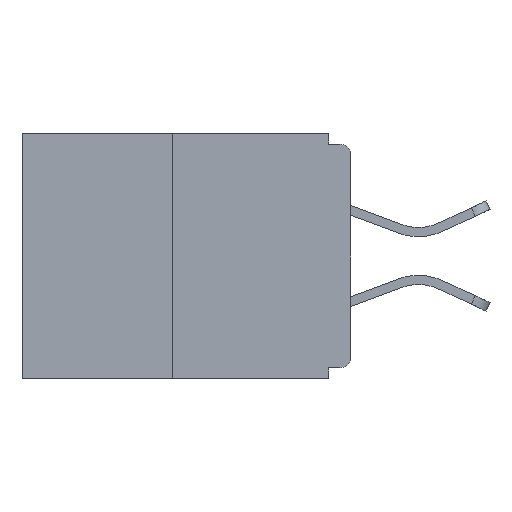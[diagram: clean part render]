
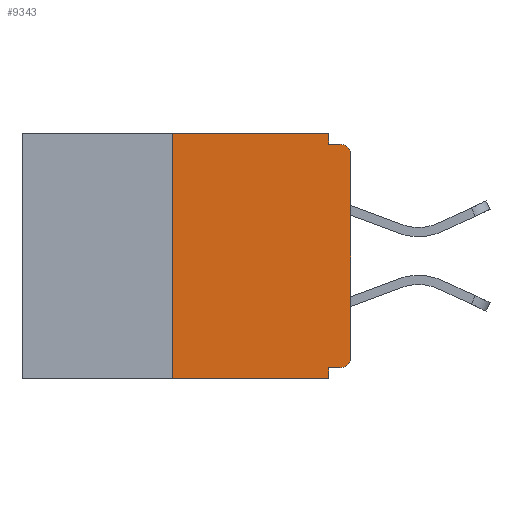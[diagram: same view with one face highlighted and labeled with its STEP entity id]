
A CAD part, left-side view. The second image highlights one B-rep face of the part: STEP entity #9343.
In plain terms, the highlighted planar face has unit normal (-1, 0, 0).
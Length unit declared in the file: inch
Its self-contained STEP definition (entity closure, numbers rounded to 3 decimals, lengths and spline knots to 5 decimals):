
#34 = DIRECTION ( 'NONE',  ( 0., -1., 0. ) ) ;
#90 = ORIENTED_EDGE ( 'NONE', *, *, #9702, .T. ) ;
#694 = CIRCLE ( 'NONE', #2859, 0.015 ) ;
#905 = FACE_OUTER_BOUND ( 'NONE', #6309, .T. ) ;
#1050 = VECTOR ( 'NONE', #14594, 39.37008 ) ;
#1052 = DIRECTION ( 'NONE',  ( 0., -1., 0. ) ) ;
#1120 = VECTOR ( 'NONE', #1052, 39.37008 ) ;
#1260 = VECTOR ( 'NONE', #14195, 39.37008 ) ;
#1294 = AXIS2_PLACEMENT_3D ( 'NONE', #4451, #4503, #5705 ) ;
#1401 = CARTESIAN_POINT ( 'NONE',  ( 0., 0.015, -0.03 ) ) ;
#1433 = LINE ( 'NONE', #3499, #1260 ) ;
#1468 = EDGE_CURVE ( 'NONE', #8898, #9207, #5351, .T. ) ;
#1534 = CIRCLE ( 'NONE', #13776, 0.015 ) ;
#1638 = CARTESIAN_POINT ( 'NONE',  ( 0., 0.015, -0.015 ) ) ;
#1789 = CARTESIAN_POINT ( 'NONE',  ( 0., 0.031, 0. ) ) ;
#1922 = VERTEX_POINT ( 'NONE', #9896 ) ;
#1983 = VECTOR ( 'NONE', #34, 39.37008 ) ;
#2243 = LINE ( 'NONE', #13547, #11268 ) ;
#2253 = ORIENTED_EDGE ( 'NONE', *, *, #13000, .F. ) ;
#2496 = EDGE_CURVE ( 'NONE', #8124, #4469, #1433, .T. ) ;
#2743 = ORIENTED_EDGE ( 'NONE', *, *, #12982, .F. ) ;
#2766 = CARTESIAN_POINT ( 'NONE',  ( 0., 0., 0. ) ) ;
#2859 = AXIS2_PLACEMENT_3D ( 'NONE', #1401, #3673, #8273 ) ;
#3013 = VECTOR ( 'NONE', #8521, 39.37008 ) ;
#3152 = ORIENTED_EDGE ( 'NONE', *, *, #2496, .F. ) ;
#3384 = CARTESIAN_POINT ( 'NONE',  ( 0., 0., -0.313 ) ) ;
#3420 = ORIENTED_EDGE ( 'NONE', *, *, #10922, .T. ) ;
#3435 = PLANE ( 'NONE',  #1294 ) ;
#3499 = CARTESIAN_POINT ( 'NONE',  ( 0., 0., -0.328 ) ) ;
#3620 = CARTESIAN_POINT ( 'NONE',  ( 0., 0.031, -0.343 ) ) ;
#3673 = DIRECTION ( 'NONE',  ( -1., 0., 0. ) ) ;
#3739 = ORIENTED_EDGE ( 'NONE', *, *, #1468, .F. ) ;
#4188 = EDGE_CURVE ( 'NONE', #8089, #10902, #6366, .T. ) ;
#4451 = CARTESIAN_POINT ( 'NONE',  ( 0., 0.46, 0. ) ) ;
#4469 = VERTEX_POINT ( 'NONE', #5397 ) ;
#4503 = DIRECTION ( 'NONE',  ( 1., 0., 0. ) ) ;
#4775 = DIRECTION ( 'NONE',  ( -1., 0., 0. ) ) ;
#5178 = CARTESIAN_POINT ( 'NONE',  ( 0., 0.031, 0. ) ) ;
#5351 = LINE ( 'NONE', #10404, #1120 ) ;
#5397 = CARTESIAN_POINT ( 'NONE',  ( 0., 0.031, -0.328 ) ) ;
#5651 = ORIENTED_EDGE ( 'NONE', *, *, #4188, .T. ) ;
#5667 = CARTESIAN_POINT ( 'NONE',  ( 0., 0., -0.03 ) ) ;
#5705 = DIRECTION ( 'NONE',  ( 0., 0., -1. ) ) ;
#6140 = CARTESIAN_POINT ( 'NONE',  ( 0., 0., -0.015 ) ) ;
#6309 = EDGE_LOOP ( 'NONE', ( #3739, #9972, #3420, #2743, #3152, #9008, #5651, #90, #2253, #8982 ) ) ;
#6366 = LINE ( 'NONE', #2766, #7252 ) ;
#6676 = CARTESIAN_POINT ( 'NONE',  ( 0., 0.25, 0. ) ) ;
#7252 = VECTOR ( 'NONE', #12063, 39.37008 ) ;
#7277 = LINE ( 'NONE', #5178, #1050 ) ;
#7494 = DIRECTION ( 'NONE',  ( 0., 0., -1. ) ) ;
#7796 = LINE ( 'NONE', #6140, #3013 ) ;
#8089 = VERTEX_POINT ( 'NONE', #3384 ) ;
#8124 = VERTEX_POINT ( 'NONE', #10945 ) ;
#8188 = LINE ( 'NONE', #13854, #1983 ) ;
#8273 = DIRECTION ( 'NONE',  ( 0., 0., -1. ) ) ;
#8521 = DIRECTION ( 'NONE',  ( 0., -1., 0. ) ) ;
#8898 = VERTEX_POINT ( 'NONE', #6676 ) ;
#8982 = ORIENTED_EDGE ( 'NONE', *, *, #9890, .F. ) ;
#9008 = ORIENTED_EDGE ( 'NONE', *, *, #12899, .T. ) ;
#9207 = VERTEX_POINT ( 'NONE', #1789 ) ;
#9343 = ADVANCED_FACE ( 'NONE', ( #905 ), #3435, .F. ) ;
#9702 = EDGE_CURVE ( 'NONE', #10902, #13835, #694, .T. ) ;
#9890 = EDGE_CURVE ( 'NONE', #9207, #10961, #7277, .T. ) ;
#9896 = CARTESIAN_POINT ( 'NONE',  ( 0., 0.25, -0.343 ) ) ;
#9972 = ORIENTED_EDGE ( 'NONE', *, *, #14562, .F. ) ;
#10404 = CARTESIAN_POINT ( 'NONE',  ( 0., 0.46, 0. ) ) ;
#10642 = DIRECTION ( 'NONE',  ( 0., 0., -1. ) ) ;
#10902 = VERTEX_POINT ( 'NONE', #5667 ) ;
#10922 = EDGE_CURVE ( 'NONE', #1922, #12936, #8188, .T. ) ;
#10945 = CARTESIAN_POINT ( 'NONE',  ( 0., 0.015, -0.328 ) ) ;
#10961 = VERTEX_POINT ( 'NONE', #14192 ) ;
#11268 = VECTOR ( 'NONE', #14718, 39.37008 ) ;
#11865 = LINE ( 'NONE', #14450, #12427 ) ;
#12063 = DIRECTION ( 'NONE',  ( 0., 0., 1. ) ) ;
#12427 = VECTOR ( 'NONE', #7494, 39.37008 ) ;
#12899 = EDGE_CURVE ( 'NONE', #8124, #8089, #1534, .T. ) ;
#12936 = VERTEX_POINT ( 'NONE', #3620 ) ;
#12982 = EDGE_CURVE ( 'NONE', #4469, #12936, #11865, .T. ) ;
#13000 = EDGE_CURVE ( 'NONE', #10961, #13835, #7796, .T. ) ;
#13547 = CARTESIAN_POINT ( 'NONE',  ( 0., 0.25, 0. ) ) ;
#13776 = AXIS2_PLACEMENT_3D ( 'NONE', #14255, #4775, #10642 ) ;
#13835 = VERTEX_POINT ( 'NONE', #1638 ) ;
#13854 = CARTESIAN_POINT ( 'NONE',  ( 0., 0.46, -0.343 ) ) ;
#14192 = CARTESIAN_POINT ( 'NONE',  ( 0., 0.031, -0.015 ) ) ;
#14195 = DIRECTION ( 'NONE',  ( 0., 1., 0. ) ) ;
#14255 = CARTESIAN_POINT ( 'NONE',  ( 0., 0.015, -0.313 ) ) ;
#14450 = CARTESIAN_POINT ( 'NONE',  ( 0., 0.031, -0.343 ) ) ;
#14562 = EDGE_CURVE ( 'NONE', #1922, #8898, #2243, .T. ) ;
#14594 = DIRECTION ( 'NONE',  ( 0., 0., -1. ) ) ;
#14718 = DIRECTION ( 'NONE',  ( 0., 0., 1. ) ) ;
